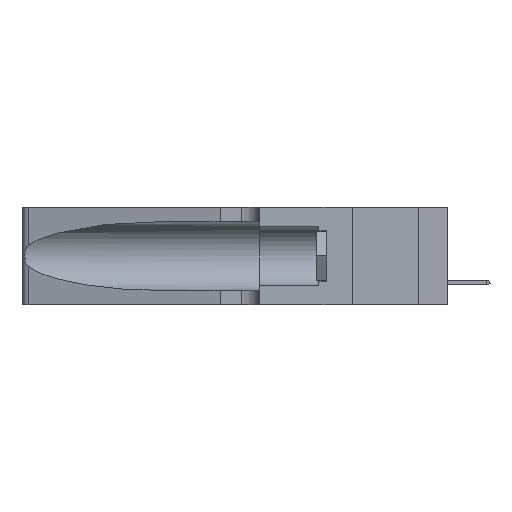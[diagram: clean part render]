
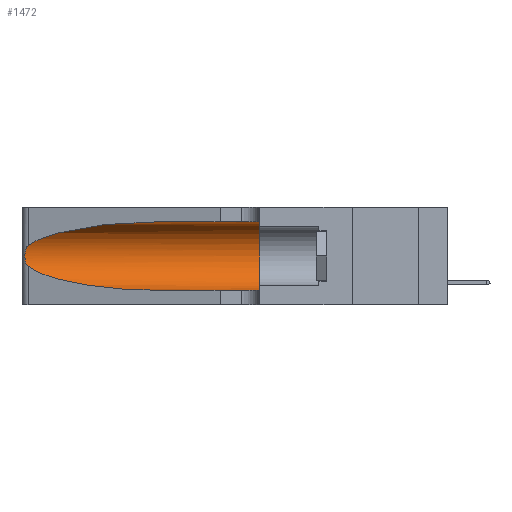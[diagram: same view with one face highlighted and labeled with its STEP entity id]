
A CAD part, left-side view. The second image highlights one B-rep face of the part: STEP entity #1472.
In plain terms, the highlighted cylindrical face has radius 3.308 mm (diameter 6.617 mm), a partial arc.
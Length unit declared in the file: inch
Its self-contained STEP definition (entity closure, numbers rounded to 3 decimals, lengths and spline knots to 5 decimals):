
#126 = CYLINDRICAL_SURFACE ( 'NONE', #2012, 0.13025 ) ;
#623 = EDGE_CURVE ( 'NONE', #11932, #8002, #9077, .T. ) ;
#1110 = ORIENTED_EDGE ( 'NONE', *, *, #3400, .T. ) ;
#1178 = CARTESIAN_POINT ( 'NONE',  ( 0.26018, 1.23835, 0.19895 ) ) ;
#1247 = CARTESIAN_POINT ( 'NONE',  ( 0.26075, 1.23896, 0.178 ) ) ;
#1472 = ADVANCED_FACE ( 'NONE', ( #2374 ), #126, .F. ) ;
#1658 = DIRECTION ( 'NONE',  ( 0., 0., -1. ) ) ;
#1780 = EDGE_CURVE ( 'NONE', #1985, #14026, #17230, .T. ) ;
#1985 = VERTEX_POINT ( 'NONE', #17527 ) ;
#2012 = AXIS2_PLACEMENT_3D ( 'NONE', #15786, #3044, #1658 ) ;
#2374 = FACE_OUTER_BOUND ( 'NONE', #17326, .T. ) ;
#2673 = CARTESIAN_POINT ( 'NONE',  ( 0.25487, 1.22718, 0.22369 ) ) ;
#2755 = CARTESIAN_POINT ( 'NONE',  ( 0.1305, 0.72297, 0.31525 ) ) ;
#2958 = EDGE_CURVE ( 'NONE', #5245, #17713, #18149, .T. ) ;
#3044 = DIRECTION ( 'NONE',  ( 0., -1., 0. ) ) ;
#3400 = EDGE_CURVE ( 'NONE', #17713, #1985, #10344, .T. ) ;
#4049 = ORIENTED_EDGE ( 'NONE', *, *, #1780, .T. ) ;
#4252 = CARTESIAN_POINT ( 'NONE',  ( 0.18966, 0.96281, 0.31525 ) ) ;
#5245 = VERTEX_POINT ( 'NONE', #2673 ) ;
#5543 = CARTESIAN_POINT ( 'NONE',  ( 0.25787, 1.23484, 0.2124 ) ) ;
#6507 = CARTESIAN_POINT ( 'NONE',  ( 0.1305, 1.61858, 0.31525 ) ) ;
#6807 =( BOUNDED_CURVE ( )  B_SPLINE_CURVE ( 3, ( #2755, #4252, #8350, #12929 ),
 .UNSPECIFIED., .F., .F. ) 
 B_SPLINE_CURVE_WITH_KNOTS ( ( 4, 4 ),
 ( 1.5708, 2.84003 ),
 .UNSPECIFIED. ) 
 CURVE ( )  GEOMETRIC_REPRESENTATION_ITEM ( )  RATIONAL_B_SPLINE_CURVE ( ( 1., 0.87, 0.87, 1. ) ) 
 REPRESENTATION_ITEM ( '' )  );
#7050 = CARTESIAN_POINT ( 'NONE',  ( 0.25854, 1.2359, 0.20912 ) ) ;
#7728 = CARTESIAN_POINT ( 'NONE',  ( 0.25487, 1.22718, 0.14631 ) ) ;
#8002 = VERTEX_POINT ( 'NONE', #16545 ) ;
#8227 = CARTESIAN_POINT ( 'NONE',  ( 0.25555, 1.22993, 0.14849 ) ) ;
#8236 = CARTESIAN_POINT ( 'NONE',  ( 0.1305, 0.35, 0.05475 ) ) ;
#8280 = CARTESIAN_POINT ( 'NONE',  ( 0.25555, 1.22994, 0.2215 ) ) ;
#8350 = CARTESIAN_POINT ( 'NONE',  ( 0.2373, 1.15595, 0.28018 ) ) ;
#8401 = CARTESIAN_POINT ( 'NONE',  ( 0.26017, 1.23833, 0.17102 ) ) ;
#8547 = CARTESIAN_POINT ( 'NONE',  ( 0.25487, 1.22718, 0.14631 ) ) ;
#8623 = VECTOR ( 'NONE', #9371, 39.37008 ) ;
#9013 = ORIENTED_EDGE ( 'NONE', *, *, #623, .F. ) ;
#9077 = LINE ( 'NONE', #6507, #8623 ) ;
#9371 = DIRECTION ( 'NONE',  ( 0., -1., 0. ) ) ;
#9598 = CARTESIAN_POINT ( 'NONE',  ( 0.25789, 1.23486, 0.15765 ) ) ;
#9751 = DIRECTION ( 'NONE',  ( 0., -1., 0. ) ) ;
#9782 = CARTESIAN_POINT ( 'NONE',  ( 0.26075, 1.23896, 0.19203 ) ) ;
#10344 =( BOUNDED_CURVE ( )  B_SPLINE_CURVE ( 3, ( #7728, #12406, #15295, #12351 ),
 .UNSPECIFIED., .F., .F. ) 
 B_SPLINE_CURVE_WITH_KNOTS ( ( 4, 4 ),
 ( 3.44316, 4.71239 ),
 .UNSPECIFIED. ) 
 CURVE ( )  GEOMETRIC_REPRESENTATION_ITEM ( )  RATIONAL_B_SPLINE_CURVE ( ( 1., 0.87, 0.87, 1. ) ) 
 REPRESENTATION_ITEM ( '' )  );
#11104 = CARTESIAN_POINT ( 'NONE',  ( 0.1305, 0.72297, 0.31525 ) ) ;
#11731 = CARTESIAN_POINT ( 'NONE',  ( 0.1305, 0.35, 0.185 ) ) ;
#11857 = VECTOR ( 'NONE', #9751, 39.37008 ) ;
#11932 = VERTEX_POINT ( 'NONE', #11104 ) ;
#12351 = CARTESIAN_POINT ( 'NONE',  ( 0.1305, 0.72297, 0.05475 ) ) ;
#12406 = CARTESIAN_POINT ( 'NONE',  ( 0.2373, 1.15595, 0.08982 ) ) ;
#12433 = CIRCLE ( 'NONE', #14099, 0.13025 ) ;
#12528 = EDGE_CURVE ( 'NONE', #8002, #14026, #12433, .T. ) ;
#12569 = CARTESIAN_POINT ( 'NONE',  ( 0.1305, 1.61858, 0.05475 ) ) ;
#12929 = CARTESIAN_POINT ( 'NONE',  ( 0.25487, 1.22718, 0.22369 ) ) ;
#13489 = ORIENTED_EDGE ( 'NONE', *, *, #2958, .T. ) ;
#13932 = CARTESIAN_POINT ( 'NONE',  ( 0.25639, 1.23184, 0.21858 ) ) ;
#14026 = VERTEX_POINT ( 'NONE', #8236 ) ;
#14061 = CARTESIAN_POINT ( 'NONE',  ( 0.25639, 1.23186, 0.15144 ) ) ;
#14099 = AXIS2_PLACEMENT_3D ( 'NONE', #11731, #15920, #17374 ) ;
#14129 = CARTESIAN_POINT ( 'NONE',  ( 0.25487, 1.22718, 0.22369 ) ) ;
#14184 = EDGE_CURVE ( 'NONE', #11932, #5245, #6807, .T. ) ;
#14187 = CARTESIAN_POINT ( 'NONE',  ( 0.25487, 1.22718, 0.14631 ) ) ;
#15295 = CARTESIAN_POINT ( 'NONE',  ( 0.18966, 0.96281, 0.05475 ) ) ;
#15786 = CARTESIAN_POINT ( 'NONE',  ( 0.1305, 1.61858, 0.185 ) ) ;
#15920 = DIRECTION ( 'NONE',  ( 0., 1., 0. ) ) ;
#16091 = ORIENTED_EDGE ( 'NONE', *, *, #14184, .T. ) ;
#16545 = CARTESIAN_POINT ( 'NONE',  ( 0.1305, 0.35, 0.31525 ) ) ;
#16981 = CARTESIAN_POINT ( 'NONE',  ( 0.25856, 1.23593, 0.16098 ) ) ;
#17230 = LINE ( 'NONE', #12569, #11857 ) ;
#17326 = EDGE_LOOP ( 'NONE', ( #16091, #13489, #1110, #4049, #18091, #9013 ) ) ;
#17374 = DIRECTION ( 'NONE',  ( 0., 0., 1. ) ) ;
#17527 = CARTESIAN_POINT ( 'NONE',  ( 0.1305, 0.72297, 0.05475 ) ) ;
#17713 = VERTEX_POINT ( 'NONE', #8547 ) ;
#18091 = ORIENTED_EDGE ( 'NONE', *, *, #12528, .F. ) ;
#18149 = B_SPLINE_CURVE_WITH_KNOTS ( 'NONE', 3,
 ( #14129, #8280, #13932, #5543, #7050, #1178, #9782, #1247, #8401, #16981, #9598, #14061, #8227, #14187 ),
 .UNSPECIFIED., .F., .F.,
 ( 4, 2, 2, 2, 2, 2, 4 ),
 ( 0., 0.00027, 0.00053, 0.00107, 0.0016, 0.00187, 0.00214 ),
 .UNSPECIFIED. ) ;
